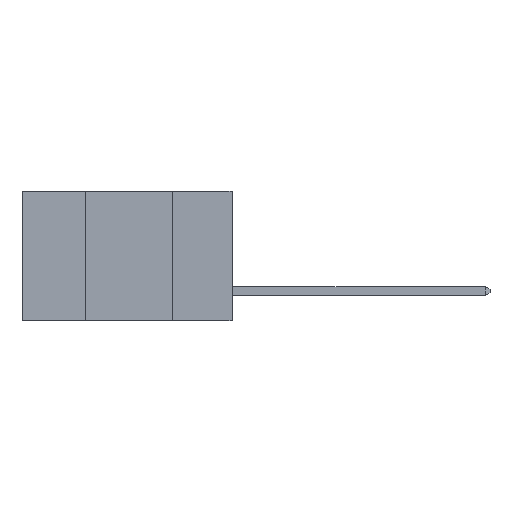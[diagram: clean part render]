
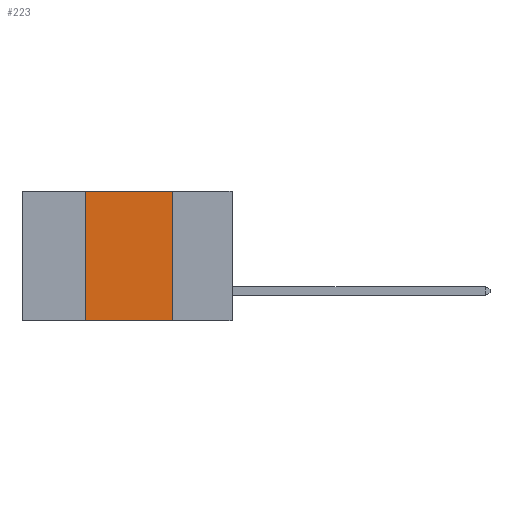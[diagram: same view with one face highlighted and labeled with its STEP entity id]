
A CAD part, left-side view. The second image highlights one B-rep face of the part: STEP entity #223.
In plain terms, the highlighted planar face has unit normal (-1, 0, 0).
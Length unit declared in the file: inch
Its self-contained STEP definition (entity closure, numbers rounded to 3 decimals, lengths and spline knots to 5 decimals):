
#192 = CARTESIAN_POINT ( 'NONE',  ( 0., 0.17, 0. ) ) ;
#223 = ADVANCED_FACE ( 'NONE', ( #14648 ), #27224, .F. ) ;
#1643 = DIRECTION ( 'NONE',  ( 0., -1., 0. ) ) ;
#6735 = CARTESIAN_POINT ( 'NONE',  ( 0., 0.17, 0. ) ) ;
#6758 = EDGE_CURVE ( 'NONE', #26014, #25867, #12352, .T. ) ;
#7946 = CARTESIAN_POINT ( 'NONE',  ( 0., 0.42, -0.37 ) ) ;
#8613 = DIRECTION ( 'NONE',  ( 0., 0., -1. ) ) ;
#9465 = EDGE_CURVE ( 'NONE', #19103, #26014, #20485, .T. ) ;
#10416 = EDGE_CURVE ( 'NONE', #13560, #25867, #18963, .T. ) ;
#10916 = ORIENTED_EDGE ( 'NONE', *, *, #9465, .F. ) ;
#12209 = DIRECTION ( 'NONE',  ( 0., 0., -1. ) ) ;
#12352 = LINE ( 'NONE', #6735, #32511 ) ;
#13560 = VERTEX_POINT ( 'NONE', #7946 ) ;
#14370 = ORIENTED_EDGE ( 'NONE', *, *, #10416, .T. ) ;
#14648 = FACE_OUTER_BOUND ( 'NONE', #25391, .T. ) ;
#14835 = AXIS2_PLACEMENT_3D ( 'NONE', #22357, #21896, #8613 ) ;
#15182 = CARTESIAN_POINT ( 'NONE',  ( 0., 0.42, 0. ) ) ;
#15967 = VECTOR ( 'NONE', #17049, 39.37008 ) ;
#16151 = VECTOR ( 'NONE', #30876, 39.37008 ) ;
#17049 = DIRECTION ( 'NONE',  ( 0., -1., 0. ) ) ;
#18752 = CARTESIAN_POINT ( 'NONE',  ( 0., 0.17, -0.37 ) ) ;
#18963 = LINE ( 'NONE', #33599, #20879 ) ;
#19103 = VERTEX_POINT ( 'NONE', #15182 ) ;
#20485 = LINE ( 'NONE', #32652, #15967 ) ;
#20879 = VECTOR ( 'NONE', #1643, 39.37008 ) ;
#21142 = EDGE_CURVE ( 'NONE', #13560, #19103, #30086, .T. ) ;
#21896 = DIRECTION ( 'NONE',  ( 1., 0., 0. ) ) ;
#22357 = CARTESIAN_POINT ( 'NONE',  ( 0., 0.6, 0. ) ) ;
#25391 = EDGE_LOOP ( 'NONE', ( #27109, #10916, #31967, #14370 ) ) ;
#25867 = VERTEX_POINT ( 'NONE', #18752 ) ;
#26014 = VERTEX_POINT ( 'NONE', #192 ) ;
#27109 = ORIENTED_EDGE ( 'NONE', *, *, #6758, .F. ) ;
#27224 = PLANE ( 'NONE',  #14835 ) ;
#28286 = CARTESIAN_POINT ( 'NONE',  ( 0., 0.42, 0. ) ) ;
#30086 = LINE ( 'NONE', #28286, #16151 ) ;
#30876 = DIRECTION ( 'NONE',  ( 0., 0., 1. ) ) ;
#31967 = ORIENTED_EDGE ( 'NONE', *, *, #21142, .F. ) ;
#32511 = VECTOR ( 'NONE', #12209, 39.37008 ) ;
#32652 = CARTESIAN_POINT ( 'NONE',  ( 0., 0.6, 0. ) ) ;
#33599 = CARTESIAN_POINT ( 'NONE',  ( 0., 0.6, -0.37 ) ) ;
